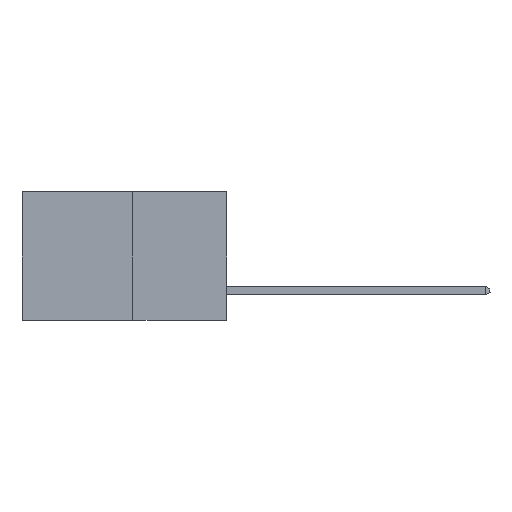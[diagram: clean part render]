
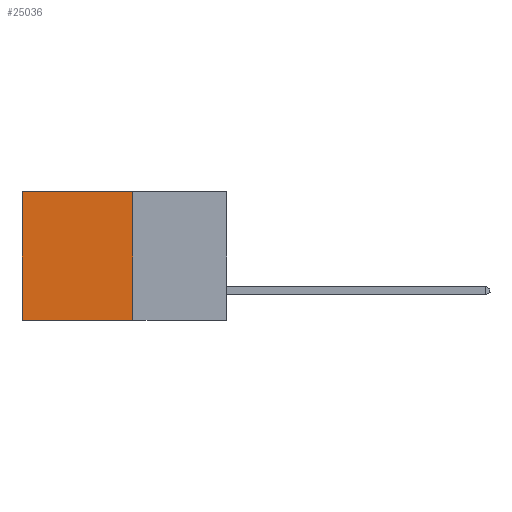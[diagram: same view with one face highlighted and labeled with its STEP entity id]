
A CAD part, left-side view. The second image highlights one B-rep face of the part: STEP entity #25036.
In plain terms, the highlighted planar face has unit normal (-1, 0, 0).
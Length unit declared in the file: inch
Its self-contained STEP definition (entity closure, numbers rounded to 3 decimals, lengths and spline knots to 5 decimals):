
#548 = CARTESIAN_POINT ( 'NONE',  ( 0.277, 0.27, 0. ) ) ;
#620 = VECTOR ( 'NONE', #22550, 39.37008 ) ;
#2278 = CARTESIAN_POINT ( 'NONE',  ( 0.277, 0.27, -0.37 ) ) ;
#2355 = LINE ( 'NONE', #6566, #27841 ) ;
#2370 = AXIS2_PLACEMENT_3D ( 'NONE', #9185, #11680, #28872 ) ;
#3083 = VERTEX_POINT ( 'NONE', #24417 ) ;
#3613 = VERTEX_POINT ( 'NONE', #22539 ) ;
#4677 = ORIENTED_EDGE ( 'NONE', *, *, #11852, .F. ) ;
#5905 = CARTESIAN_POINT ( 'NONE',  ( 0.277, 0.59, -0.37 ) ) ;
#6315 = VECTOR ( 'NONE', #22861, 39.37008 ) ;
#6566 = CARTESIAN_POINT ( 'NONE',  ( 0.277, 0.59, -0.37 ) ) ;
#6679 = DIRECTION ( 'NONE',  ( 0., 0., -1. ) ) ;
#7581 = EDGE_CURVE ( 'NONE', #3083, #15971, #26772, .T. ) ;
#8557 = EDGE_CURVE ( 'NONE', #15971, #29397, #2355, .T. ) ;
#9185 = CARTESIAN_POINT ( 'NONE',  ( 0.277, 0.27, -0.37 ) ) ;
#11601 = LINE ( 'NONE', #2278, #17424 ) ;
#11680 = DIRECTION ( 'NONE',  ( 1., 0., 0. ) ) ;
#11852 = EDGE_CURVE ( 'NONE', #3613, #29397, #14603, .T. ) ;
#13277 = EDGE_LOOP ( 'NONE', ( #23887, #4677, #24944, #25626 ) ) ;
#14603 = LINE ( 'NONE', #17613, #620 ) ;
#15971 = VERTEX_POINT ( 'NONE', #26111 ) ;
#17424 = VECTOR ( 'NONE', #27005, 39.37008 ) ;
#17613 = CARTESIAN_POINT ( 'NONE',  ( 0.277, 0.27, -0.37 ) ) ;
#22539 = CARTESIAN_POINT ( 'NONE',  ( 0.277, 0.27, -0.37 ) ) ;
#22550 = DIRECTION ( 'NONE',  ( 0., 1., 0. ) ) ;
#22861 = DIRECTION ( 'NONE',  ( 0., 1., 0. ) ) ;
#23887 = ORIENTED_EDGE ( 'NONE', *, *, #8557, .T. ) ;
#23998 = PLANE ( 'NONE',  #2370 ) ;
#24417 = CARTESIAN_POINT ( 'NONE',  ( 0.277, 0.27, 0. ) ) ;
#24944 = ORIENTED_EDGE ( 'NONE', *, *, #26441, .F. ) ;
#25036 = ADVANCED_FACE ( 'NONE', ( #28627 ), #23998, .F. ) ;
#25626 = ORIENTED_EDGE ( 'NONE', *, *, #7581, .T. ) ;
#26111 = CARTESIAN_POINT ( 'NONE',  ( 0.277, 0.59, 0. ) ) ;
#26441 = EDGE_CURVE ( 'NONE', #3083, #3613, #11601, .T. ) ;
#26772 = LINE ( 'NONE', #548, #6315 ) ;
#27005 = DIRECTION ( 'NONE',  ( 0., 0., -1. ) ) ;
#27841 = VECTOR ( 'NONE', #6679, 39.37008 ) ;
#28627 = FACE_OUTER_BOUND ( 'NONE', #13277, .T. ) ;
#28872 = DIRECTION ( 'NONE',  ( 0., 0., -1. ) ) ;
#29397 = VERTEX_POINT ( 'NONE', #5905 ) ;
